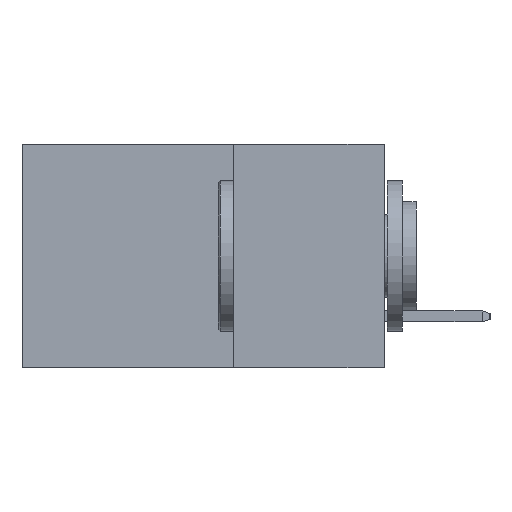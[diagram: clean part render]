
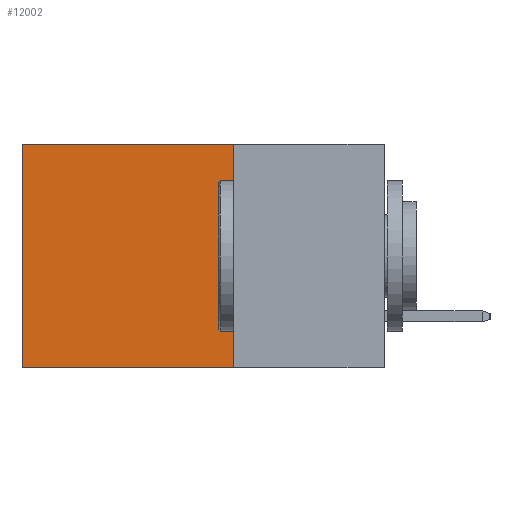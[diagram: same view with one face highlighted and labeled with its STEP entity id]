
A CAD part, left-side view. The second image highlights one B-rep face of the part: STEP entity #12002.
In plain terms, the highlighted planar face has unit normal (-1, 0, 0).
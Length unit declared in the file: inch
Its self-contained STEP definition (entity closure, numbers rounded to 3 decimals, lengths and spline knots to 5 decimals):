
#179 = CARTESIAN_POINT ( 'NONE',  ( 0.2615, 0.25, -0.37 ) ) ;
#449 = CARTESIAN_POINT ( 'NONE',  ( 0.2615, 0.25, -0.37 ) ) ;
#469 = EDGE_CURVE ( 'NONE', #3660, #9893, #12797, .T. ) ;
#711 = CARTESIAN_POINT ( 'NONE',  ( 0.2615, 0.6, 0. ) ) ;
#1267 = EDGE_CURVE ( 'NONE', #11482, #9893, #7039, .T. ) ;
#1352 = VECTOR ( 'NONE', #2666, 39.37008 ) ;
#1526 = FACE_OUTER_BOUND ( 'NONE', #9533, .T. ) ;
#1798 = EDGE_CURVE ( 'NONE', #10734, #11482, #3162, .T. ) ;
#2266 = ORIENTED_EDGE ( 'NONE', *, *, #1267, .T. ) ;
#2513 = CARTESIAN_POINT ( 'NONE',  ( 0.2615, 0.6, -0.37 ) ) ;
#2666 = DIRECTION ( 'NONE',  ( 0., 1., 0. ) ) ;
#2858 = CARTESIAN_POINT ( 'NONE',  ( 0.2615, 0.25, -0.37 ) ) ;
#2896 = DIRECTION ( 'NONE',  ( 0., 0., -1. ) ) ;
#3003 = AXIS2_PLACEMENT_3D ( 'NONE', #179, #12073, #5566 ) ;
#3162 = LINE ( 'NONE', #9921, #6037 ) ;
#3296 = CARTESIAN_POINT ( 'NONE',  ( 0.2615, 0.6, -0.37 ) ) ;
#3419 = ORIENTED_EDGE ( 'NONE', *, *, #8315, .F. ) ;
#3660 = VERTEX_POINT ( 'NONE', #2858 ) ;
#3952 = DIRECTION ( 'NONE',  ( 0., 0., -1. ) ) ;
#5566 = DIRECTION ( 'NONE',  ( 0., 0., -1. ) ) ;
#6037 = VECTOR ( 'NONE', #12517, 39.37008 ) ;
#6789 = CARTESIAN_POINT ( 'NONE',  ( 0.2615, 0.25, 0. ) ) ;
#7039 = LINE ( 'NONE', #2513, #12778 ) ;
#7926 = LINE ( 'NONE', #10442, #13277 ) ;
#8315 = EDGE_CURVE ( 'NONE', #10734, #3660, #7926, .T. ) ;
#9533 = EDGE_LOOP ( 'NONE', ( #2266, #12811, #3419, #13055 ) ) ;
#9893 = VERTEX_POINT ( 'NONE', #3296 ) ;
#9921 = CARTESIAN_POINT ( 'NONE',  ( 0.2615, 0.25, 0. ) ) ;
#10442 = CARTESIAN_POINT ( 'NONE',  ( 0.2615, 0.25, -0.37 ) ) ;
#10734 = VERTEX_POINT ( 'NONE', #6789 ) ;
#10988 = PLANE ( 'NONE',  #3003 ) ;
#11482 = VERTEX_POINT ( 'NONE', #711 ) ;
#12002 = ADVANCED_FACE ( 'NONE', ( #1526 ), #10988, .F. ) ;
#12073 = DIRECTION ( 'NONE',  ( 1., 0., 0. ) ) ;
#12517 = DIRECTION ( 'NONE',  ( 0., 1., 0. ) ) ;
#12778 = VECTOR ( 'NONE', #3952, 39.37008 ) ;
#12797 = LINE ( 'NONE', #449, #1352 ) ;
#12811 = ORIENTED_EDGE ( 'NONE', *, *, #469, .F. ) ;
#13055 = ORIENTED_EDGE ( 'NONE', *, *, #1798, .T. ) ;
#13277 = VECTOR ( 'NONE', #2896, 39.37008 ) ;
